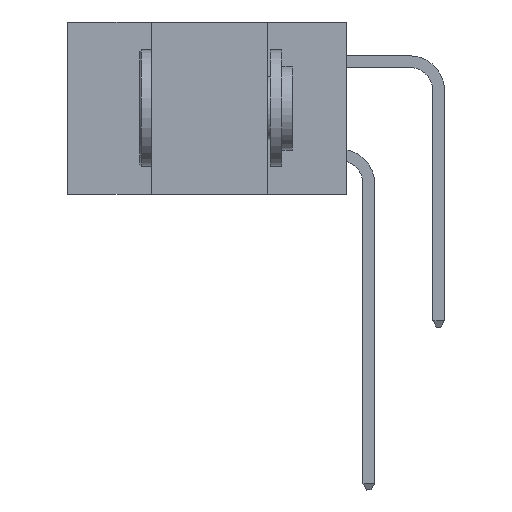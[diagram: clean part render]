
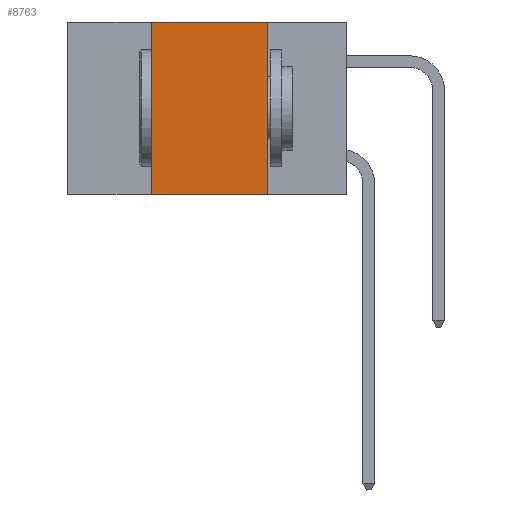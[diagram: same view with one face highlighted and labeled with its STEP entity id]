
A CAD part, left-side view. The second image highlights one B-rep face of the part: STEP entity #8763.
In plain terms, the highlighted planar face has unit normal (-1, 0, 0).
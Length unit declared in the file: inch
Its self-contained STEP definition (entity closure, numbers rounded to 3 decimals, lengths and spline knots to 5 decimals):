
#212 = LINE ( 'NONE', #2687, #5271 ) ;
#284 = VECTOR ( 'NONE', #9400, 39.37008 ) ;
#296 = CARTESIAN_POINT ( 'NONE',  ( 0., 0.42, 0. ) ) ;
#1398 = VERTEX_POINT ( 'NONE', #1688 ) ;
#1688 = CARTESIAN_POINT ( 'NONE',  ( 0., 0.17, 0. ) ) ;
#2010 = EDGE_CURVE ( 'NONE', #4865, #1398, #5223, .T. ) ;
#2687 = CARTESIAN_POINT ( 'NONE',  ( 0., 0.6, -0.37 ) ) ;
#2803 = CARTESIAN_POINT ( 'NONE',  ( 0., 0.17, 0. ) ) ;
#3223 = CARTESIAN_POINT ( 'NONE',  ( 0., 0.6, 0. ) ) ;
#3857 = ORIENTED_EDGE ( 'NONE', *, *, #11340, .F. ) ;
#4665 = CARTESIAN_POINT ( 'NONE',  ( 0., 0.42, -0.37 ) ) ;
#4708 = DIRECTION ( 'NONE',  ( 1., 0., 0. ) ) ;
#4812 = CARTESIAN_POINT ( 'NONE',  ( 0., 0.17, -0.37 ) ) ;
#4865 = VERTEX_POINT ( 'NONE', #9902 ) ;
#5141 = DIRECTION ( 'NONE',  ( 0., -1., 0. ) ) ;
#5223 = LINE ( 'NONE', #3223, #9300 ) ;
#5271 = VECTOR ( 'NONE', #5535, 39.37008 ) ;
#5535 = DIRECTION ( 'NONE',  ( 0., -1., 0. ) ) ;
#5562 = LINE ( 'NONE', #2803, #7470 ) ;
#6254 = EDGE_LOOP ( 'NONE', ( #3857, #9355, #13840, #14479 ) ) ;
#6658 = VERTEX_POINT ( 'NONE', #4812 ) ;
#6799 = EDGE_CURVE ( 'NONE', #8713, #4865, #12803, .T. ) ;
#6847 = PLANE ( 'NONE',  #10286 ) ;
#7470 = VECTOR ( 'NONE', #14045, 39.37008 ) ;
#8713 = VERTEX_POINT ( 'NONE', #4665 ) ;
#8763 = ADVANCED_FACE ( 'NONE', ( #11699 ), #6847, .F. ) ;
#9265 = EDGE_CURVE ( 'NONE', #8713, #6658, #212, .T. ) ;
#9300 = VECTOR ( 'NONE', #5141, 39.37008 ) ;
#9355 = ORIENTED_EDGE ( 'NONE', *, *, #2010, .F. ) ;
#9400 = DIRECTION ( 'NONE',  ( 0., 0., 1. ) ) ;
#9902 = CARTESIAN_POINT ( 'NONE',  ( 0., 0.42, 0. ) ) ;
#10286 = AXIS2_PLACEMENT_3D ( 'NONE', #11528, #4708, #10385 ) ;
#10385 = DIRECTION ( 'NONE',  ( 0., 0., -1. ) ) ;
#11340 = EDGE_CURVE ( 'NONE', #1398, #6658, #5562, .T. ) ;
#11528 = CARTESIAN_POINT ( 'NONE',  ( 0., 0.6, 0. ) ) ;
#11699 = FACE_OUTER_BOUND ( 'NONE', #6254, .T. ) ;
#12803 = LINE ( 'NONE', #296, #284 ) ;
#13840 = ORIENTED_EDGE ( 'NONE', *, *, #6799, .F. ) ;
#14045 = DIRECTION ( 'NONE',  ( 0., 0., -1. ) ) ;
#14479 = ORIENTED_EDGE ( 'NONE', *, *, #9265, .T. ) ;
